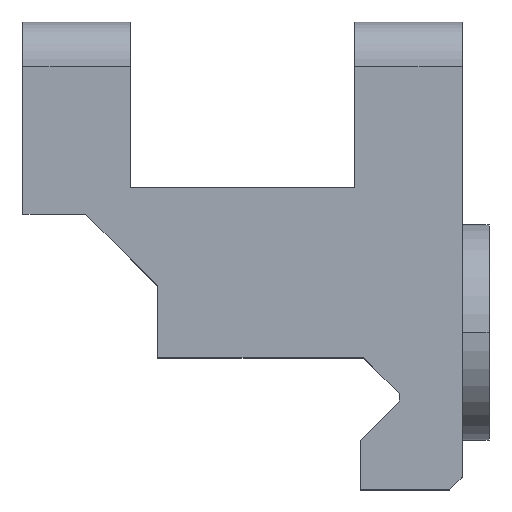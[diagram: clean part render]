
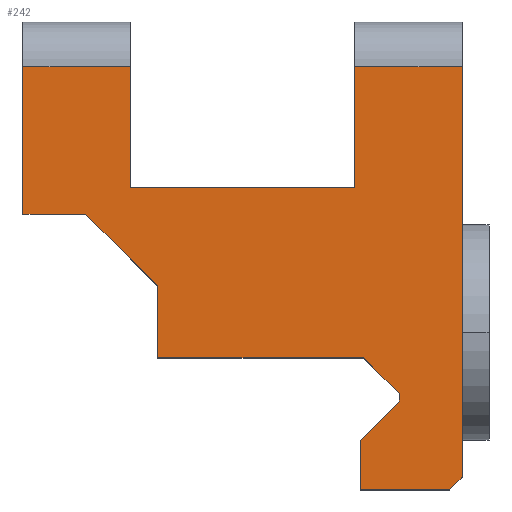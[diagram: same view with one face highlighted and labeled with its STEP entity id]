
A CAD part, top view. The second image highlights one B-rep face of the part: STEP entity #242.
In plain terms, the highlighted planar face has unit normal (0, 0, 1).
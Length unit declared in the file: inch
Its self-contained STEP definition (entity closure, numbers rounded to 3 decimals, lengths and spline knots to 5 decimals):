
#4 = VECTOR ( 'NONE', #1743, 39.37008 ) ;
#18 = ORIENTED_EDGE ( 'NONE', *, *, #1507, .T. ) ;
#20 = EDGE_CURVE ( 'NONE', #842, #535, #54, .T. ) ;
#26 = VERTEX_POINT ( 'NONE', #814 ) ;
#32 = VECTOR ( 'NONE', #390, 39.37008 ) ;
#40 = CARTESIAN_POINT ( 'NONE',  ( 0.5925, 0.18082, 0.6 ) ) ;
#43 = DIRECTION ( 'NONE',  ( 0., 0., 1. ) ) ;
#45 = CARTESIAN_POINT ( 'NONE',  ( -0.63025, 0.92, 0.6 ) ) ;
#48 = ORIENTED_EDGE ( 'NONE', *, *, #20, .T. ) ;
#54 = LINE ( 'NONE', #1480, #1503 ) ;
#55 = DIRECTION ( 'NONE',  ( -0.707, 0.707, 0. ) ) ;
#58 = LINE ( 'NONE', #1512, #1351 ) ;
#74 = CARTESIAN_POINT ( 'NONE',  ( 0.4175, 0.0105, 0.6 ) ) ;
#80 = LINE ( 'NONE', #629, #852 ) ;
#88 = CARTESIAN_POINT ( 'NONE',  ( 0.4175, 0.0105, 0.6 ) ) ;
#94 = CARTESIAN_POINT ( 'NONE',  ( 0.5925, 0.92, 0.6 ) ) ;
#99 = LINE ( 'NONE', #1584, #1097 ) ;
#116 = ORIENTED_EDGE ( 'NONE', *, *, #838, .T. ) ;
#140 = ORIENTED_EDGE ( 'NONE', *, *, #1388, .T. ) ;
#151 = FACE_OUTER_BOUND ( 'NONE', #1550, .T. ) ;
#155 = VECTOR ( 'NONE', #475, 39.37008 ) ;
#169 = VECTOR ( 'NONE', #1755, 39.37008 ) ;
#177 = VECTOR ( 'NONE', #1169, 39.37008 ) ;
#180 = CARTESIAN_POINT ( 'NONE',  ( 0., 0., 0.6 ) ) ;
#183 = ORIENTED_EDGE ( 'NONE', *, *, #1759, .T. ) ;
#185 = CARTESIAN_POINT ( 'NONE',  ( 0.3085, -0.1195, 0.6 ) ) ;
#187 = ORIENTED_EDGE ( 'NONE', *, *, #1679, .T. ) ;
#223 = CARTESIAN_POINT ( 'NONE',  ( -0.45525, 0.51, 0.6 ) ) ;
#225 = DIRECTION ( 'NONE',  ( 0., -1., 0. ) ) ;
#241 = DIRECTION ( 'NONE',  ( 0., -1., 0. ) ) ;
#242 = ADVANCED_FACE ( 'NONE', ( #151 ), #1395, .T. ) ;
#254 = VERTEX_POINT ( 'NONE', #185 ) ;
#267 = VERTEX_POINT ( 'NONE', #1132 ) ;
#299 = CARTESIAN_POINT ( 'NONE',  ( 0.4175, -0.0105, 0.6 ) ) ;
#305 = LINE ( 'NONE', #745, #155 ) ;
#327 = DIRECTION ( 'NONE',  ( 0., 1., 0. ) ) ;
#351 = DIRECTION ( 'NONE',  ( 1., 0., 0. ) ) ;
#354 = ORIENTED_EDGE ( 'NONE', *, *, #1752, .T. ) ;
#357 = ORIENTED_EDGE ( 'NONE', *, *, #504, .T. ) ;
#384 = CARTESIAN_POINT ( 'NONE',  ( -0.45525, 0.51, 0.6 ) ) ;
#390 = DIRECTION ( 'NONE',  ( 0., -1., 0. ) ) ;
#455 = EDGE_CURVE ( 'NONE', #524, #1088, #698, .T. ) ;
#475 = DIRECTION ( 'NONE',  ( 0., -1., 0. ) ) ;
#494 = ORIENTED_EDGE ( 'NONE', *, *, #1585, .T. ) ;
#504 = EDGE_CURVE ( 'NONE', #26, #1014, #99, .T. ) ;
#506 = DIRECTION ( 'NONE',  ( 0., -1., 0. ) ) ;
#515 = CARTESIAN_POINT ( 'NONE',  ( -0.33138, 0.585, 0.6 ) ) ;
#523 = VERTEX_POINT ( 'NONE', #515 ) ;
#524 = VERTEX_POINT ( 'NONE', #1036 ) ;
#535 = VERTEX_POINT ( 'NONE', #94 ) ;
#549 = VERTEX_POINT ( 'NONE', #1596 ) ;
#576 = ORIENTED_EDGE ( 'NONE', *, *, #1692, .T. ) ;
#602 = LINE ( 'NONE', #45, #1083 ) ;
#608 = VERTEX_POINT ( 'NONE', #1085 ) ;
#616 = VERTEX_POINT ( 'NONE', #646 ) ;
#617 = EDGE_CURVE ( 'NONE', #876, #842, #1343, .T. ) ;
#629 = CARTESIAN_POINT ( 'NONE',  ( -0.45525, 0.585, 0.6 ) ) ;
#646 = CARTESIAN_POINT ( 'NONE',  ( 0.4175, -0.0105, 0.6 ) ) ;
#684 = VERTEX_POINT ( 'NONE', #1488 ) ;
#698 = LINE ( 'NONE', #384, #4 ) ;
#745 = CARTESIAN_POINT ( 'NONE',  ( 0.3085, -0.1195, 0.6 ) ) ;
#805 = LINE ( 'NONE', #1390, #1176 ) ;
#812 = LINE ( 'NONE', #1451, #32 ) ;
#814 = CARTESIAN_POINT ( 'NONE',  ( -0.25525, 0.11, 0.6 ) ) ;
#821 = DIRECTION ( 'NONE',  ( 0., 1., 0. ) ) ;
#826 = AXIS2_PLACEMENT_3D ( 'NONE', #180, #43, #1529 ) ;
#838 = EDGE_CURVE ( 'NONE', #616, #254, #1476, .T. ) ;
#842 = VERTEX_POINT ( 'NONE', #40 ) ;
#851 = ORIENTED_EDGE ( 'NONE', *, *, #872, .F. ) ;
#852 = VECTOR ( 'NONE', #1043, 39.37008 ) ;
#868 = VECTOR ( 'NONE', #351, 39.37008 ) ;
#872 = EDGE_CURVE ( 'NONE', #684, #1088, #805, .T. ) ;
#876 = VERTEX_POINT ( 'NONE', #980 ) ;
#882 = LINE ( 'NONE', #1044, #1579 ) ;
#891 = LINE ( 'NONE', #1300, #1244 ) ;
#894 = CARTESIAN_POINT ( 'NONE',  ( 0.318, 0.11, 0.6 ) ) ;
#912 = ORIENTED_EDGE ( 'NONE', *, *, #455, .T. ) ;
#949 = DIRECTION ( 'NONE',  ( 0.707, 0.707, 0. ) ) ;
#965 = DIRECTION ( 'NONE',  ( -1., 0., 0. ) ) ;
#970 = LINE ( 'NONE', #894, #177 ) ;
#980 = CARTESIAN_POINT ( 'NONE',  ( 0.5925, -0.22164, 0.6 ) ) ;
#1014 = VERTEX_POINT ( 'NONE', #1705 ) ;
#1024 = CARTESIAN_POINT ( 'NONE',  ( -0.33138, 0.92, 0.6 ) ) ;
#1036 = CARTESIAN_POINT ( 'NONE',  ( -0.63025, 0.51, 0.6 ) ) ;
#1041 = ORIENTED_EDGE ( 'NONE', *, *, #1729, .F. ) ;
#1043 = DIRECTION ( 'NONE',  ( 1., 0., 0. ) ) ;
#1044 = CARTESIAN_POINT ( 'NONE',  ( 0.55714, -0.257, 0.6 ) ) ;
#1057 = DIRECTION ( 'NONE',  ( 1., 0., 0. ) ) ;
#1058 = LINE ( 'NONE', #1133, #1677 ) ;
#1071 = VERTEX_POINT ( 'NONE', #1024 ) ;
#1083 = VECTOR ( 'NONE', #1534, 39.37008 ) ;
#1084 = CARTESIAN_POINT ( 'NONE',  ( 0.29362, 0.585, 0.6 ) ) ;
#1085 = CARTESIAN_POINT ( 'NONE',  ( 0.55714, -0.257, 0.6 ) ) ;
#1088 = VERTEX_POINT ( 'NONE', #223 ) ;
#1097 = VECTOR ( 'NONE', #1057, 39.37008 ) ;
#1098 = VERTEX_POINT ( 'NONE', #74 ) ;
#1116 = ORIENTED_EDGE ( 'NONE', *, *, #1572, .T. ) ;
#1124 = VECTOR ( 'NONE', #506, 39.37008 ) ;
#1132 = CARTESIAN_POINT ( 'NONE',  ( 0.3085, -0.257, 0.6 ) ) ;
#1133 = CARTESIAN_POINT ( 'NONE',  ( -0.33138, 0.585, 0.6 ) ) ;
#1169 = DIRECTION ( 'NONE',  ( 0.707, -0.707, 0. ) ) ;
#1176 = VECTOR ( 'NONE', #55, 39.37008 ) ;
#1189 = ORIENTED_EDGE ( 'NONE', *, *, #1242, .T. ) ;
#1228 = LINE ( 'NONE', #1554, #868 ) ;
#1242 = EDGE_CURVE ( 'NONE', #608, #876, #882, .T. ) ;
#1244 = VECTOR ( 'NONE', #225, 39.37008 ) ;
#1266 = LINE ( 'NONE', #88, #1124 ) ;
#1300 = CARTESIAN_POINT ( 'NONE',  ( -0.63025, 0.51, 0.6 ) ) ;
#1343 = LINE ( 'NONE', #1495, #169 ) ;
#1351 = VECTOR ( 'NONE', #965, 39.37008 ) ;
#1387 = VERTEX_POINT ( 'NONE', #1084 ) ;
#1388 = EDGE_CURVE ( 'NONE', #535, #1602, #58, .T. ) ;
#1390 = CARTESIAN_POINT ( 'NONE',  ( -0.45525, 0.51, 0.6 ) ) ;
#1395 = PLANE ( 'NONE',  #826 ) ;
#1403 = CARTESIAN_POINT ( 'NONE',  ( 0.29362, 0.92, 0.6 ) ) ;
#1451 = CARTESIAN_POINT ( 'NONE',  ( 0.29362, 0.585, 0.6 ) ) ;
#1466 = ORIENTED_EDGE ( 'NONE', *, *, #1654, .T. ) ;
#1476 = LINE ( 'NONE', #299, #1535 ) ;
#1480 = CARTESIAN_POINT ( 'NONE',  ( 0.5925, -0.22164, 0.6 ) ) ;
#1488 = CARTESIAN_POINT ( 'NONE',  ( -0.25525, 0.31, 0.6 ) ) ;
#1495 = CARTESIAN_POINT ( 'NONE',  ( 0.5925, -0.22164, 0.6 ) ) ;
#1503 = VECTOR ( 'NONE', #821, 39.37008 ) ;
#1506 = DIRECTION ( 'NONE',  ( -0.707, -0.707, 0. ) ) ;
#1507 = EDGE_CURVE ( 'NONE', #523, #1071, #1058, .T. ) ;
#1512 = CARTESIAN_POINT ( 'NONE',  ( 0.29362, 0.92, 0.6 ) ) ;
#1523 = EDGE_CURVE ( 'NONE', #1071, #549, #602, .T. ) ;
#1529 = DIRECTION ( 'NONE',  ( 1., 0., 0. ) ) ;
#1534 = DIRECTION ( 'NONE',  ( -1., 0., 0. ) ) ;
#1535 = VECTOR ( 'NONE', #1506, 39.37008 ) ;
#1550 = EDGE_LOOP ( 'NONE', ( #48, #140, #183, #1041, #18, #1775, #576, #912, #851, #187, #357, #1466, #354, #116, #494, #1116, #1189, #1614 ) ) ;
#1554 = CARTESIAN_POINT ( 'NONE',  ( 0.3085, -0.257, 0.6 ) ) ;
#1561 = CARTESIAN_POINT ( 'NONE',  ( -0.25525, 0.31, 0.6 ) ) ;
#1572 = EDGE_CURVE ( 'NONE', #267, #608, #1228, .T. ) ;
#1579 = VECTOR ( 'NONE', #949, 39.37008 ) ;
#1584 = CARTESIAN_POINT ( 'NONE',  ( 0.318, 0.11, 0.6 ) ) ;
#1585 = EDGE_CURVE ( 'NONE', #254, #267, #305, .T. ) ;
#1596 = CARTESIAN_POINT ( 'NONE',  ( -0.63025, 0.92, 0.6 ) ) ;
#1602 = VERTEX_POINT ( 'NONE', #1403 ) ;
#1614 = ORIENTED_EDGE ( 'NONE', *, *, #617, .T. ) ;
#1617 = LINE ( 'NONE', #1561, #1636 ) ;
#1636 = VECTOR ( 'NONE', #241, 39.37008 ) ;
#1654 = EDGE_CURVE ( 'NONE', #1014, #1098, #970, .T. ) ;
#1677 = VECTOR ( 'NONE', #327, 39.37008 ) ;
#1679 = EDGE_CURVE ( 'NONE', #684, #26, #1617, .T. ) ;
#1692 = EDGE_CURVE ( 'NONE', #549, #524, #891, .T. ) ;
#1705 = CARTESIAN_POINT ( 'NONE',  ( 0.318, 0.11, 0.6 ) ) ;
#1729 = EDGE_CURVE ( 'NONE', #523, #1387, #80, .T. ) ;
#1743 = DIRECTION ( 'NONE',  ( 1., 0., 0. ) ) ;
#1752 = EDGE_CURVE ( 'NONE', #1098, #616, #1266, .T. ) ;
#1755 = DIRECTION ( 'NONE',  ( 0., 1., 0. ) ) ;
#1759 = EDGE_CURVE ( 'NONE', #1602, #1387, #812, .T. ) ;
#1775 = ORIENTED_EDGE ( 'NONE', *, *, #1523, .T. ) ;
